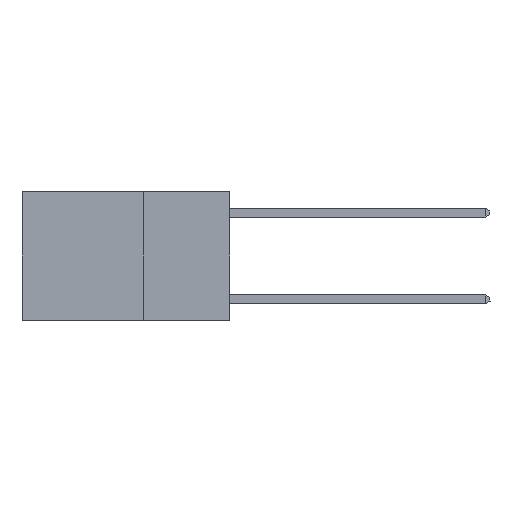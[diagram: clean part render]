
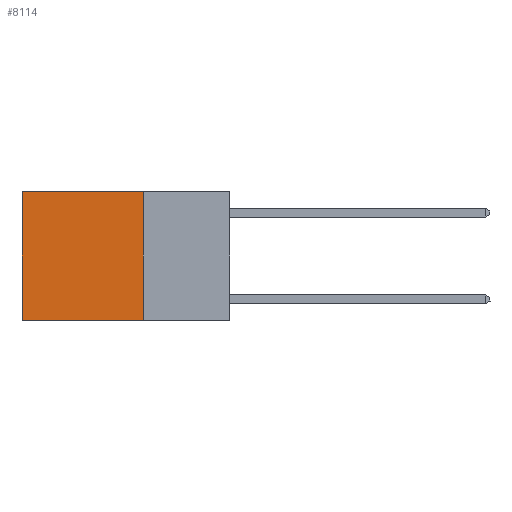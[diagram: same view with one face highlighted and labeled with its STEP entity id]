
A CAD part, left-side view. The second image highlights one B-rep face of the part: STEP entity #8114.
In plain terms, the highlighted planar face has unit normal (-1, 0, 0).
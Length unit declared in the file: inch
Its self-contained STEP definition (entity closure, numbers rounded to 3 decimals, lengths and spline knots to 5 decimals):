
#736 = EDGE_CURVE ( 'NONE', #7049, #11855, #18253, .T. ) ;
#903 = LINE ( 'NONE', #18296, #12994 ) ;
#911 = AXIS2_PLACEMENT_3D ( 'NONE', #5090, #17307, #3475 ) ;
#1503 = VERTEX_POINT ( 'NONE', #17500 ) ;
#1908 = DIRECTION ( 'NONE',  ( 0., 0., -1. ) ) ;
#2462 = DIRECTION ( 'NONE',  ( 0., 0., -1. ) ) ;
#2580 = ORIENTED_EDGE ( 'NONE', *, *, #21445, .T. ) ;
#2674 = ORIENTED_EDGE ( 'NONE', *, *, #736, .F. ) ;
#2941 = VECTOR ( 'NONE', #3036, 39.37008 ) ;
#3036 = DIRECTION ( 'NONE',  ( 0., 1., 0. ) ) ;
#3475 = DIRECTION ( 'NONE',  ( 0., 0., -1. ) ) ;
#3482 = CARTESIAN_POINT ( 'NONE',  ( 0.2625, 0.25, 0. ) ) ;
#4518 = VECTOR ( 'NONE', #8654, 39.37008 ) ;
#4556 = CARTESIAN_POINT ( 'NONE',  ( 0.2625, 0.6, -0.37 ) ) ;
#4861 = LINE ( 'NONE', #10692, #13354 ) ;
#5090 = CARTESIAN_POINT ( 'NONE',  ( 0.2625, 0.25, 0. ) ) ;
#7049 = VERTEX_POINT ( 'NONE', #22300 ) ;
#8114 = ADVANCED_FACE ( 'NONE', ( #22674 ), #10485, .F. ) ;
#8654 = DIRECTION ( 'NONE',  ( 0., 1., 0. ) ) ;
#10485 = PLANE ( 'NONE',  #911 ) ;
#10692 = CARTESIAN_POINT ( 'NONE',  ( 0.2625, 0.25, 0. ) ) ;
#11494 = EDGE_CURVE ( 'NONE', #12968, #1503, #22778, .T. ) ;
#11855 = VERTEX_POINT ( 'NONE', #4556 ) ;
#11966 = EDGE_CURVE ( 'NONE', #12968, #7049, #4861, .T. ) ;
#12968 = VERTEX_POINT ( 'NONE', #3482 ) ;
#12994 = VECTOR ( 'NONE', #2462, 39.37008 ) ;
#13354 = VECTOR ( 'NONE', #1908, 39.37008 ) ;
#13829 = ORIENTED_EDGE ( 'NONE', *, *, #11494, .T. ) ;
#14144 = CARTESIAN_POINT ( 'NONE',  ( 0.2625, 0.25, -0.37 ) ) ;
#17307 = DIRECTION ( 'NONE',  ( 1., 0., 0. ) ) ;
#17500 = CARTESIAN_POINT ( 'NONE',  ( 0.2625, 0.6, 0. ) ) ;
#18253 = LINE ( 'NONE', #14144, #4518 ) ;
#18296 = CARTESIAN_POINT ( 'NONE',  ( 0.2625, 0.6, 0. ) ) ;
#21278 = ORIENTED_EDGE ( 'NONE', *, *, #11966, .F. ) ;
#21445 = EDGE_CURVE ( 'NONE', #1503, #11855, #903, .T. ) ;
#21688 = EDGE_LOOP ( 'NONE', ( #2580, #2674, #21278, #13829 ) ) ;
#22300 = CARTESIAN_POINT ( 'NONE',  ( 0.2625, 0.25, -0.37 ) ) ;
#22490 = CARTESIAN_POINT ( 'NONE',  ( 0.2625, 0.25, 0. ) ) ;
#22674 = FACE_OUTER_BOUND ( 'NONE', #21688, .T. ) ;
#22778 = LINE ( 'NONE', #22490, #2941 ) ;
